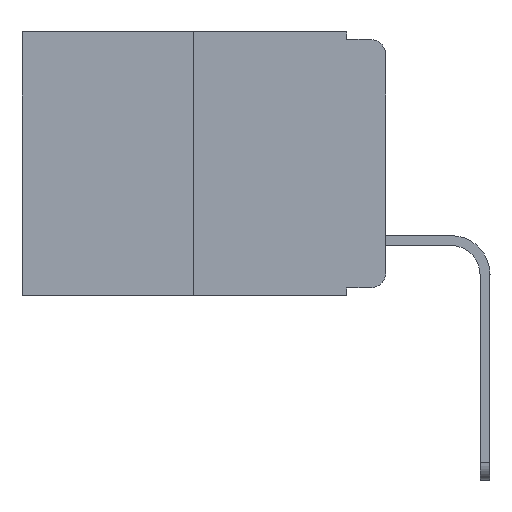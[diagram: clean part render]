
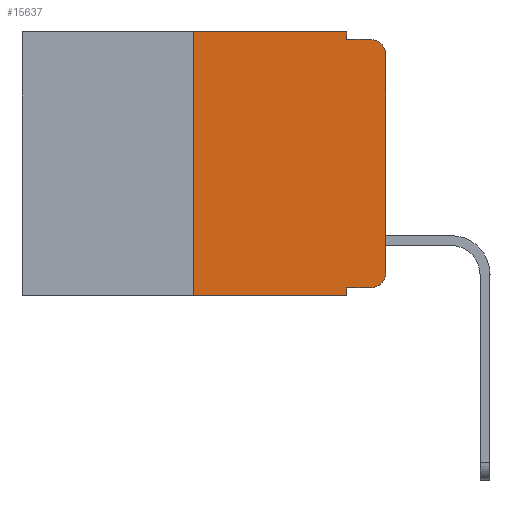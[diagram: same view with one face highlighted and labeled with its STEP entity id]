
A CAD part, left-side view. The second image highlights one B-rep face of the part: STEP entity #15637.
In plain terms, the highlighted planar face has unit normal (-1, 0, 0).
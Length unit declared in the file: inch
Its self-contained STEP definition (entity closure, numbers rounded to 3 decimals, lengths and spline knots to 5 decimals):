
#1 = VERTEX_POINT ( 'NONE', #22815 ) ;
#231 = VERTEX_POINT ( 'NONE', #19050 ) ;
#348 = VECTOR ( 'NONE', #19455, 39.37008 ) ;
#1075 = CARTESIAN_POINT ( 'NONE',  ( 0., 0.051, -0.333 ) ) ;
#1223 = EDGE_CURVE ( 'NONE', #231, #5754, #2349, .T. ) ;
#1306 = CARTESIAN_POINT ( 'NONE',  ( 0., 0.051, -0.01 ) ) ;
#1738 = EDGE_CURVE ( 'NONE', #5114, #7774, #12551, .T. ) ;
#1901 = ORIENTED_EDGE ( 'NONE', *, *, #6590, .F. ) ;
#2140 = CARTESIAN_POINT ( 'NONE',  ( 0., 0.473, 0. ) ) ;
#2349 = CIRCLE ( 'NONE', #7065, 0.02 ) ;
#3029 = LINE ( 'NONE', #4143, #21604 ) ;
#3197 = LINE ( 'NONE', #1306, #15411 ) ;
#3228 = ORIENTED_EDGE ( 'NONE', *, *, #18271, .F. ) ;
#3948 = DIRECTION ( 'NONE',  ( 0., 0., -1. ) ) ;
#4053 = AXIS2_PLACEMENT_3D ( 'NONE', #5901, #18947, #5744 ) ;
#4143 = CARTESIAN_POINT ( 'NONE',  ( 0., 0.25, 0. ) ) ;
#5114 = VERTEX_POINT ( 'NONE', #16048 ) ;
#5437 = CARTESIAN_POINT ( 'NONE',  ( 0., 0., -0.313 ) ) ;
#5578 = VERTEX_POINT ( 'NONE', #16485 ) ;
#5744 = DIRECTION ( 'NONE',  ( 0., 0., -1. ) ) ;
#5754 = VERTEX_POINT ( 'NONE', #12834 ) ;
#5901 = CARTESIAN_POINT ( 'NONE',  ( 0., 0.02, -0.313 ) ) ;
#6217 = ORIENTED_EDGE ( 'NONE', *, *, #1223, .T. ) ;
#6590 = EDGE_CURVE ( 'NONE', #8575, #16854, #3029, .T. ) ;
#6601 = DIRECTION ( 'NONE',  ( 0., 0., -1. ) ) ;
#6703 = VECTOR ( 'NONE', #6601, 39.37008 ) ;
#6843 = VECTOR ( 'NONE', #7513, 39.37008 ) ;
#7065 = AXIS2_PLACEMENT_3D ( 'NONE', #12451, #12532, #21685 ) ;
#7360 = CARTESIAN_POINT ( 'NONE',  ( 0., 0.473, -0.343 ) ) ;
#7513 = DIRECTION ( 'NONE',  ( 0., -1., 0. ) ) ;
#7681 = PLANE ( 'NONE',  #11542 ) ;
#7774 = VERTEX_POINT ( 'NONE', #23806 ) ;
#8072 = CIRCLE ( 'NONE', #4053, 0.02 ) ;
#8233 = CARTESIAN_POINT ( 'NONE',  ( 0., 0.051, 0. ) ) ;
#8575 = VERTEX_POINT ( 'NONE', #11406 ) ;
#8795 = LINE ( 'NONE', #15571, #348 ) ;
#8897 = DIRECTION ( 'NONE',  ( 0., -1., 0. ) ) ;
#9143 = CARTESIAN_POINT ( 'NONE',  ( 0., 0.051, -0.343 ) ) ;
#11279 = ORIENTED_EDGE ( 'NONE', *, *, #15944, .T. ) ;
#11406 = CARTESIAN_POINT ( 'NONE',  ( 0., 0.25, -0.343 ) ) ;
#11542 = AXIS2_PLACEMENT_3D ( 'NONE', #2140, #20580, #3948 ) ;
#11560 = ORIENTED_EDGE ( 'NONE', *, *, #1738, .T. ) ;
#11569 = EDGE_CURVE ( 'NONE', #23365, #231, #8795, .T. ) ;
#11828 = EDGE_CURVE ( 'NONE', #8575, #23115, #21226, .T. ) ;
#11844 = DIRECTION ( 'NONE',  ( 0., 0., 1. ) ) ;
#12451 = CARTESIAN_POINT ( 'NONE',  ( 0., 0.02, -0.03 ) ) ;
#12532 = DIRECTION ( 'NONE',  ( -1., 0., 0. ) ) ;
#12551 = LINE ( 'NONE', #1075, #23272 ) ;
#12834 = CARTESIAN_POINT ( 'NONE',  ( 0., 0.02, -0.01 ) ) ;
#12911 = ORIENTED_EDGE ( 'NONE', *, *, #11569, .T. ) ;
#14295 = DIRECTION ( 'NONE',  ( 0., -1., 0. ) ) ;
#14789 = EDGE_CURVE ( 'NONE', #5114, #23115, #21777, .T. ) ;
#14835 = ORIENTED_EDGE ( 'NONE', *, *, #18780, .F. ) ;
#15163 = VECTOR ( 'NONE', #8897, 39.37008 ) ;
#15411 = VECTOR ( 'NONE', #14295, 39.37008 ) ;
#15571 = CARTESIAN_POINT ( 'NONE',  ( 0., 0., 0. ) ) ;
#15637 = ADVANCED_FACE ( 'NONE', ( #20839 ), #7681, .F. ) ;
#15805 = LINE ( 'NONE', #17628, #16410 ) ;
#15944 = EDGE_CURVE ( 'NONE', #7774, #23365, #8072, .T. ) ;
#16048 = CARTESIAN_POINT ( 'NONE',  ( 0., 0.051, -0.333 ) ) ;
#16410 = VECTOR ( 'NONE', #19167, 39.37008 ) ;
#16431 = LINE ( 'NONE', #18637, #6843 ) ;
#16485 = CARTESIAN_POINT ( 'NONE',  ( 0., 0.051, -0.01 ) ) ;
#16854 = VERTEX_POINT ( 'NONE', #23101 ) ;
#16986 = ORIENTED_EDGE ( 'NONE', *, *, #21807, .F. ) ;
#17628 = CARTESIAN_POINT ( 'NONE',  ( 0., 0.051, 0. ) ) ;
#18254 = EDGE_LOOP ( 'NONE', ( #12911, #6217, #16986, #14835, #3228, #1901, #23926, #20722, #11560, #11279 ) ) ;
#18271 = EDGE_CURVE ( 'NONE', #16854, #1, #16431, .T. ) ;
#18637 = CARTESIAN_POINT ( 'NONE',  ( 0., 0.473, 0. ) ) ;
#18780 = EDGE_CURVE ( 'NONE', #1, #5578, #15805, .T. ) ;
#18947 = DIRECTION ( 'NONE',  ( -1., 0., 0. ) ) ;
#19050 = CARTESIAN_POINT ( 'NONE',  ( 0., 0., -0.03 ) ) ;
#19167 = DIRECTION ( 'NONE',  ( 0., 0., -1. ) ) ;
#19455 = DIRECTION ( 'NONE',  ( 0., 0., 1. ) ) ;
#19940 = DIRECTION ( 'NONE',  ( 0., -1., 0. ) ) ;
#20580 = DIRECTION ( 'NONE',  ( 1., 0., 0. ) ) ;
#20722 = ORIENTED_EDGE ( 'NONE', *, *, #14789, .F. ) ;
#20839 = FACE_OUTER_BOUND ( 'NONE', #18254, .T. ) ;
#21226 = LINE ( 'NONE', #7360, #15163 ) ;
#21604 = VECTOR ( 'NONE', #11844, 39.37008 ) ;
#21685 = DIRECTION ( 'NONE',  ( 0., 0., -1. ) ) ;
#21777 = LINE ( 'NONE', #8233, #6703 ) ;
#21807 = EDGE_CURVE ( 'NONE', #5578, #5754, #3197, .T. ) ;
#22815 = CARTESIAN_POINT ( 'NONE',  ( 0., 0.051, 0. ) ) ;
#23101 = CARTESIAN_POINT ( 'NONE',  ( 0., 0.25, 0. ) ) ;
#23115 = VERTEX_POINT ( 'NONE', #9143 ) ;
#23272 = VECTOR ( 'NONE', #19940, 39.37008 ) ;
#23365 = VERTEX_POINT ( 'NONE', #5437 ) ;
#23806 = CARTESIAN_POINT ( 'NONE',  ( 0., 0.02, -0.333 ) ) ;
#23926 = ORIENTED_EDGE ( 'NONE', *, *, #11828, .T. ) ;
